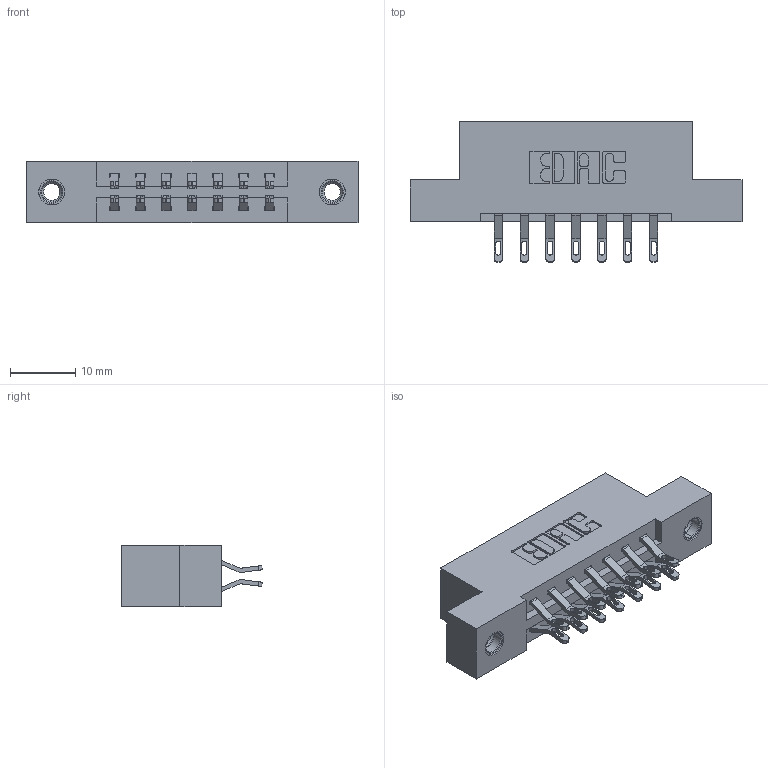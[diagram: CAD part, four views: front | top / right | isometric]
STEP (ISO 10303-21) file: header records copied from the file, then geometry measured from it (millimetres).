
FILE_DESCRIPTION (( 'STEP AP203' ), '1' );
FILE_NAME ('387-014-555-207.STEP', '2019-10-15T21:47:55', ( '' ), ( '' ), 'SwSTEP 2.0', 'SolidWorks 2016', '' );
FILE_SCHEMA (( 'CONFIG_CONTROL_DESIGN' ));
Length unit declared in the file: inch
Products named in the file (4): 345-292-001_555 Tail; 387-014-555-207; 337 Part_Flush Mounting Lugs - 0.156 Dia-TI; 345-250-001_345-250-005-103
Assembly tree (17 placements, depth 2):
  387-014-555-207
    337 Part_Flush Mounting Lugs - 0.156 Dia-TI
    345-292-001_555 Tail  x14
    345-250-001_345-250-005-103  x2
Bounding box: 50.75 x 21.47 x 9.4 mm (x, y, z)
Volume: 4909.6 mm3; surface area: 5399.3 mm2
Topology: 17 solids, 17 shells, 1014 faces, 3093 edges, 2054 vertices
Faces by surface type: plane 606, cylinder 392, cone 12, torus 4
Entity records: 11466 total; most frequent: CARTESIAN_POINT 1975, ORIENTED_EDGE 1874, DIRECTION 1747, EDGE_CURVE 937, VECTOR 769, LINE 769, VERTEX_POINT 620, AXIS2_PLACEMENT_3D 489
